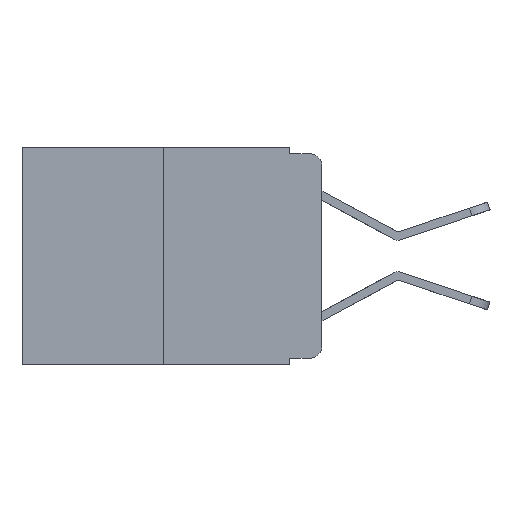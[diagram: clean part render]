
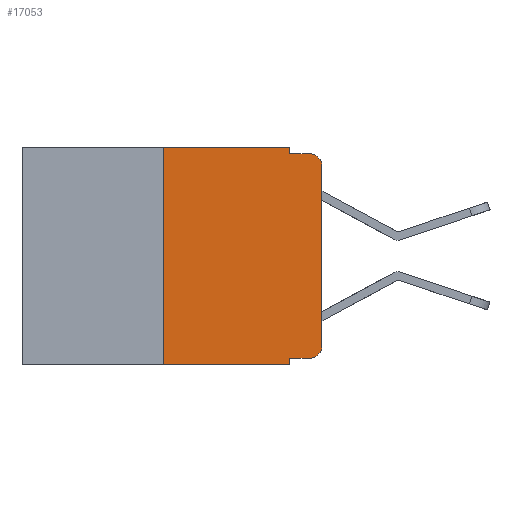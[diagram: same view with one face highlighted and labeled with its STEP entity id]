
A CAD part, left-side view. The second image highlights one B-rep face of the part: STEP entity #17053.
In plain terms, the highlighted planar face has unit normal (-1, 0, 0).
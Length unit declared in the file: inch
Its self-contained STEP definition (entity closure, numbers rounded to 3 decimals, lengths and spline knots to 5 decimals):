
#44 = DIRECTION ( 'NONE',  ( 0., 0., 1. ) ) ;
#48 = DIRECTION ( 'NONE',  ( -1., 0., 0. ) ) ;
#127 = ORIENTED_EDGE ( 'NONE', *, *, #18082, .T. ) ;
#362 = AXIS2_PLACEMENT_3D ( 'NONE', #7698, #17468, #9144 ) ;
#1164 = DIRECTION ( 'NONE',  ( 0., -1., 0. ) ) ;
#1339 = CARTESIAN_POINT ( 'NONE',  ( 0., 0., -0.03 ) ) ;
#1680 = ORIENTED_EDGE ( 'NONE', *, *, #16580, .F. ) ;
#1804 = CIRCLE ( 'NONE', #3038, 0.02 ) ;
#2166 = VERTEX_POINT ( 'NONE', #2934 ) ;
#2248 = VECTOR ( 'NONE', #5084, 39.37008 ) ;
#2319 = VECTOR ( 'NONE', #18311, 39.37008 ) ;
#2820 = ORIENTED_EDGE ( 'NONE', *, *, #7898, .T. ) ;
#2827 = CARTESIAN_POINT ( 'NONE',  ( 0., 0.02, -0.01 ) ) ;
#2934 = CARTESIAN_POINT ( 'NONE',  ( 0., 0.051, -0.333 ) ) ;
#3038 = AXIS2_PLACEMENT_3D ( 'NONE', #8686, #48, #10121 ) ;
#3290 = FACE_OUTER_BOUND ( 'NONE', #8410, .T. ) ;
#3592 = DIRECTION ( 'NONE',  ( 0., -1., 0. ) ) ;
#3707 = LINE ( 'NONE', #15715, #17819 ) ;
#3807 = VERTEX_POINT ( 'NONE', #4234 ) ;
#3817 = LINE ( 'NONE', #15957, #11439 ) ;
#4055 = VECTOR ( 'NONE', #16803, 39.37008 ) ;
#4234 = CARTESIAN_POINT ( 'NONE',  ( 0., 0., -0.313 ) ) ;
#4416 = EDGE_CURVE ( 'NONE', #3807, #11912, #3707, .T. ) ;
#4494 = VECTOR ( 'NONE', #1164, 39.37008 ) ;
#4605 = VERTEX_POINT ( 'NONE', #14640 ) ;
#5084 = DIRECTION ( 'NONE',  ( 0., 0., -1. ) ) ;
#5175 = DIRECTION ( 'NONE',  ( 1., 0., 0. ) ) ;
#5625 = ORIENTED_EDGE ( 'NONE', *, *, #15434, .T. ) ;
#5699 = LINE ( 'NONE', #12749, #2319 ) ;
#5749 = ORIENTED_EDGE ( 'NONE', *, *, #11046, .F. ) ;
#5928 = VERTEX_POINT ( 'NONE', #2827 ) ;
#6061 = LINE ( 'NONE', #17675, #2248 ) ;
#6121 = VERTEX_POINT ( 'NONE', #8775 ) ;
#6696 = VECTOR ( 'NONE', #3592, 39.37008 ) ;
#7464 = VERTEX_POINT ( 'NONE', #11750 ) ;
#7577 = DIRECTION ( 'NONE',  ( 0., 0., -1. ) ) ;
#7698 = CARTESIAN_POINT ( 'NONE',  ( 0., 0.02, -0.03 ) ) ;
#7898 = EDGE_CURVE ( 'NONE', #6121, #7464, #15347, .T. ) ;
#8153 = EDGE_CURVE ( 'NONE', #4605, #10628, #3817, .T. ) ;
#8393 = CARTESIAN_POINT ( 'NONE',  ( 0., 0.473, -0.343 ) ) ;
#8410 = EDGE_LOOP ( 'NONE', ( #9590, #127, #1680, #8690, #9539, #10434, #2820, #5749, #5625, #10512 ) ) ;
#8533 = AXIS2_PLACEMENT_3D ( 'NONE', #10880, #5175, #15065 ) ;
#8659 = EDGE_CURVE ( 'NONE', #9068, #3807, #1804, .T. ) ;
#8684 = CARTESIAN_POINT ( 'NONE',  ( 0., 0.25, 0. ) ) ;
#8686 = CARTESIAN_POINT ( 'NONE',  ( 0., 0.02, -0.313 ) ) ;
#8690 = ORIENTED_EDGE ( 'NONE', *, *, #8153, .F. ) ;
#8775 = CARTESIAN_POINT ( 'NONE',  ( 0., 0.25, -0.343 ) ) ;
#9068 = VERTEX_POINT ( 'NONE', #17860 ) ;
#9144 = DIRECTION ( 'NONE',  ( 0., 0., -1. ) ) ;
#9539 = ORIENTED_EDGE ( 'NONE', *, *, #11635, .F. ) ;
#9590 = ORIENTED_EDGE ( 'NONE', *, *, #4416, .T. ) ;
#9985 = VERTEX_POINT ( 'NONE', #11172 ) ;
#10121 = DIRECTION ( 'NONE',  ( 0., 0., -1. ) ) ;
#10434 = ORIENTED_EDGE ( 'NONE', *, *, #12568, .F. ) ;
#10512 = ORIENTED_EDGE ( 'NONE', *, *, #8659, .T. ) ;
#10628 = VERTEX_POINT ( 'NONE', #15472 ) ;
#10755 = CARTESIAN_POINT ( 'NONE',  ( 0., 0.473, 0. ) ) ;
#10880 = CARTESIAN_POINT ( 'NONE',  ( 0., 0.473, 0. ) ) ;
#10946 = LINE ( 'NONE', #10755, #6696 ) ;
#11046 = EDGE_CURVE ( 'NONE', #2166, #7464, #6061, .T. ) ;
#11172 = CARTESIAN_POINT ( 'NONE',  ( 0., 0.25, 0. ) ) ;
#11187 = CARTESIAN_POINT ( 'NONE',  ( 0., 0.051, -0.01 ) ) ;
#11439 = VECTOR ( 'NONE', #7577, 39.37008 ) ;
#11635 = EDGE_CURVE ( 'NONE', #9985, #4605, #10946, .T. ) ;
#11750 = CARTESIAN_POINT ( 'NONE',  ( 0., 0.051, -0.343 ) ) ;
#11912 = VERTEX_POINT ( 'NONE', #1339 ) ;
#12568 = EDGE_CURVE ( 'NONE', #6121, #9985, #14185, .T. ) ;
#12749 = CARTESIAN_POINT ( 'NONE',  ( 0., 0.051, -0.333 ) ) ;
#13665 = PLANE ( 'NONE',  #8533 ) ;
#14185 = LINE ( 'NONE', #8684, #14617 ) ;
#14617 = VECTOR ( 'NONE', #44, 39.37008 ) ;
#14640 = CARTESIAN_POINT ( 'NONE',  ( 0., 0.051, 0. ) ) ;
#15065 = DIRECTION ( 'NONE',  ( 0., 0., -1. ) ) ;
#15228 = CIRCLE ( 'NONE', #362, 0.02 ) ;
#15347 = LINE ( 'NONE', #8393, #4055 ) ;
#15434 = EDGE_CURVE ( 'NONE', #2166, #9068, #5699, .T. ) ;
#15472 = CARTESIAN_POINT ( 'NONE',  ( 0., 0.051, -0.01 ) ) ;
#15523 = DIRECTION ( 'NONE',  ( 0., 0., 1. ) ) ;
#15715 = CARTESIAN_POINT ( 'NONE',  ( 0., 0., 0. ) ) ;
#15957 = CARTESIAN_POINT ( 'NONE',  ( 0., 0.051, 0. ) ) ;
#16198 = LINE ( 'NONE', #11187, #4494 ) ;
#16580 = EDGE_CURVE ( 'NONE', #10628, #5928, #16198, .T. ) ;
#16803 = DIRECTION ( 'NONE',  ( 0., -1., 0. ) ) ;
#17053 = ADVANCED_FACE ( 'NONE', ( #3290 ), #13665, .F. ) ;
#17468 = DIRECTION ( 'NONE',  ( -1., 0., 0. ) ) ;
#17675 = CARTESIAN_POINT ( 'NONE',  ( 0., 0.051, 0. ) ) ;
#17819 = VECTOR ( 'NONE', #15523, 39.37008 ) ;
#17860 = CARTESIAN_POINT ( 'NONE',  ( 0., 0.02, -0.333 ) ) ;
#18082 = EDGE_CURVE ( 'NONE', #11912, #5928, #15228, .T. ) ;
#18311 = DIRECTION ( 'NONE',  ( 0., -1., 0. ) ) ;
